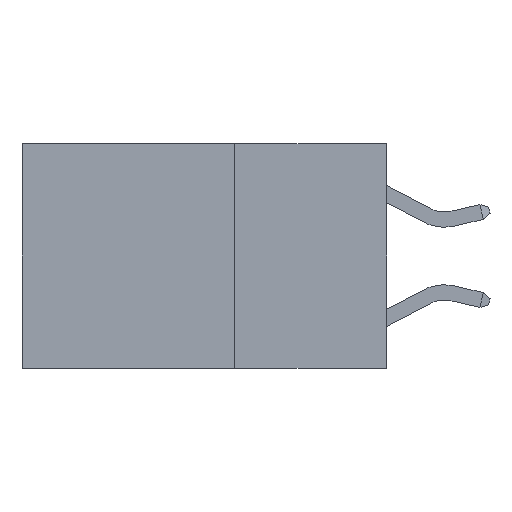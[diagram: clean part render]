
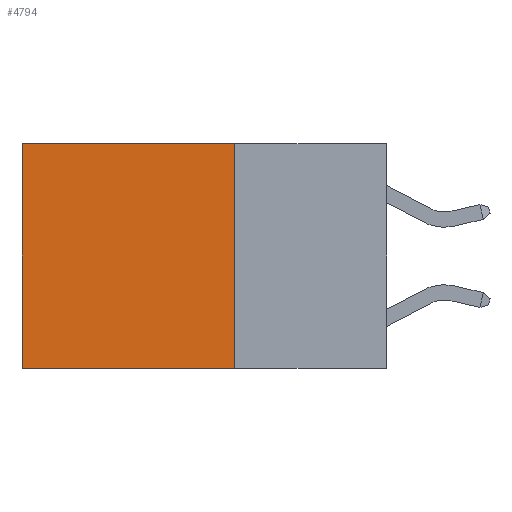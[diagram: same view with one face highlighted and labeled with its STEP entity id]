
A CAD part, left-side view. The second image highlights one B-rep face of the part: STEP entity #4794.
In plain terms, the highlighted planar face has unit normal (-1, 0, 0).
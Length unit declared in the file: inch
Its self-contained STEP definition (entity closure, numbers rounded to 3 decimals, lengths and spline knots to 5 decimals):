
#198 = VECTOR ( 'NONE', #7265, 39.37008 ) ;
#317 = DIRECTION ( 'NONE',  ( 0., 1., 0. ) ) ;
#710 = CARTESIAN_POINT ( 'NONE',  ( 0.2625, 0.25, 0. ) ) ;
#1095 = CARTESIAN_POINT ( 'NONE',  ( 0.2625, 0.6, 0. ) ) ;
#1368 = CARTESIAN_POINT ( 'NONE',  ( 0.2625, 0.6, 0. ) ) ;
#1446 = CARTESIAN_POINT ( 'NONE',  ( 0.2625, 0.6, -0.37 ) ) ;
#1759 = CARTESIAN_POINT ( 'NONE',  ( 0.2625, 0.25, 0. ) ) ;
#1874 = VECTOR ( 'NONE', #3263, 39.37008 ) ;
#1878 = LINE ( 'NONE', #1095, #198 ) ;
#2055 = LINE ( 'NONE', #4445, #4844 ) ;
#2353 = LINE ( 'NONE', #2411, #3326 ) ;
#2391 = ORIENTED_EDGE ( 'NONE', *, *, #10581, .T. ) ;
#2411 = CARTESIAN_POINT ( 'NONE',  ( 0.2625, 0.25, 0. ) ) ;
#2594 = VERTEX_POINT ( 'NONE', #7366 ) ;
#3263 = DIRECTION ( 'NONE',  ( 0., 1., 0. ) ) ;
#3326 = VECTOR ( 'NONE', #5060, 39.37008 ) ;
#3953 = ORIENTED_EDGE ( 'NONE', *, *, #4697, .T. ) ;
#4152 = CARTESIAN_POINT ( 'NONE',  ( 0.2625, 0.25, -0.37 ) ) ;
#4445 = CARTESIAN_POINT ( 'NONE',  ( 0.2625, 0.25, 0. ) ) ;
#4697 = EDGE_CURVE ( 'NONE', #9971, #6199, #2055, .T. ) ;
#4794 = ADVANCED_FACE ( 'NONE', ( #7953 ), #10557, .F. ) ;
#4844 = VECTOR ( 'NONE', #317, 39.37008 ) ;
#5060 = DIRECTION ( 'NONE',  ( 0., 0., -1. ) ) ;
#6199 = VERTEX_POINT ( 'NONE', #1368 ) ;
#6390 = EDGE_CURVE ( 'NONE', #2594, #8933, #10931, .T. ) ;
#6508 = DIRECTION ( 'NONE',  ( 0., 0., -1. ) ) ;
#7265 = DIRECTION ( 'NONE',  ( 0., 0., -1. ) ) ;
#7366 = CARTESIAN_POINT ( 'NONE',  ( 0.2625, 0.25, -0.37 ) ) ;
#7953 = FACE_OUTER_BOUND ( 'NONE', #9489, .T. ) ;
#8933 = VERTEX_POINT ( 'NONE', #1446 ) ;
#9211 = ORIENTED_EDGE ( 'NONE', *, *, #6390, .F. ) ;
#9489 = EDGE_LOOP ( 'NONE', ( #2391, #9211, #9581, #3953 ) ) ;
#9581 = ORIENTED_EDGE ( 'NONE', *, *, #10719, .F. ) ;
#9971 = VERTEX_POINT ( 'NONE', #1759 ) ;
#10557 = PLANE ( 'NONE',  #10938 ) ;
#10581 = EDGE_CURVE ( 'NONE', #6199, #8933, #1878, .T. ) ;
#10674 = DIRECTION ( 'NONE',  ( 1., 0., 0. ) ) ;
#10719 = EDGE_CURVE ( 'NONE', #9971, #2594, #2353, .T. ) ;
#10931 = LINE ( 'NONE', #4152, #1874 ) ;
#10938 = AXIS2_PLACEMENT_3D ( 'NONE', #710, #10674, #6508 ) ;
